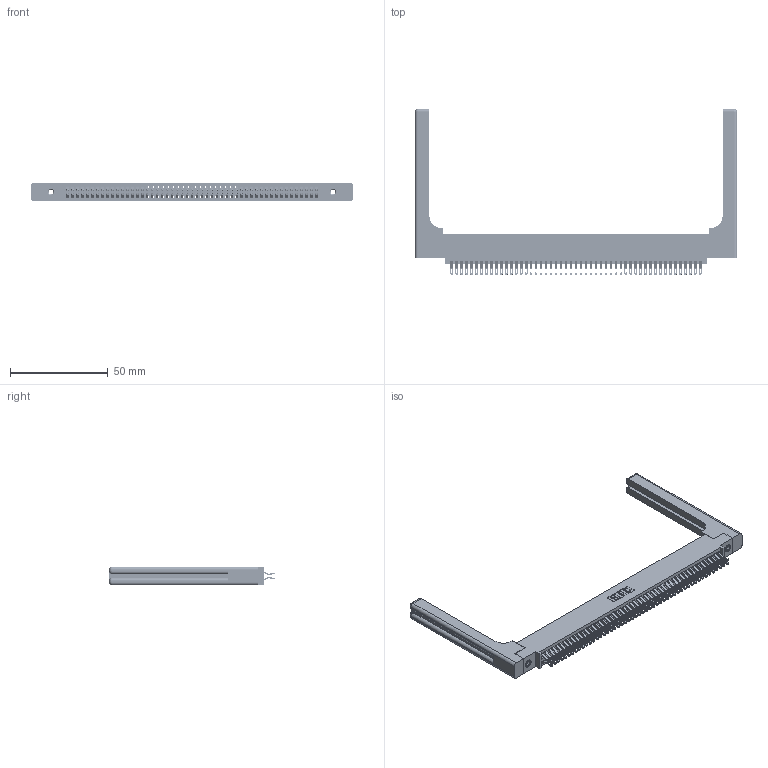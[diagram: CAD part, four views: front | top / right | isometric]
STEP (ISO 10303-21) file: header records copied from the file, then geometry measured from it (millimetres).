
FILE_DESCRIPTION (( 'STEP AP203' ), '1' );
FILE_NAME ('395-102-555-558.STEP', '2019-10-26T18:56:08', ( '' ), ( '' ), 'SwSTEP 2.0', 'SolidWorks 2016', '' );
FILE_SCHEMA (( 'CONFIG_CONTROL_DESIGN' ));
Length unit declared in the file: inch
Products named in the file (5): 345-220-058_345-220-058; 395-102-555-558; 345 Part_0.110 Offset - 0.156 Dia-TH; 345-292-001_555 Tail; 345-250-001_345-250-001-102
Assembly tree (107 placements, depth 2):
  395-102-555-558
    345 Part_0.110 Offset - 0.156 Dia-TH
    345-292-001_555 Tail  x102
    345-250-001_345-250-001-102  x2
    345-220-058_345-220-058  x2
Bounding box: 164.57 x 84.89 x 9.4 mm (x, y, z)
Volume: 24767.3 mm3; surface area: 30437.6 mm2
Topology: 107 solids, 107 shells, 6098 faces, 19073 edges, 12694 vertices
Faces by surface type: plane 3394, cylinder 2644, bspline 36, cone 12, sphere 8, torus 4
Entity records: 44444 total; most frequent: CARTESIAN_POINT 8471, ORIENTED_EDGE 7172, DIRECTION 6358, EDGE_CURVE 3586, LINE 3138, VECTOR 3138, VERTEX_POINT 2382, AXIS2_PLACEMENT_3D 1610
